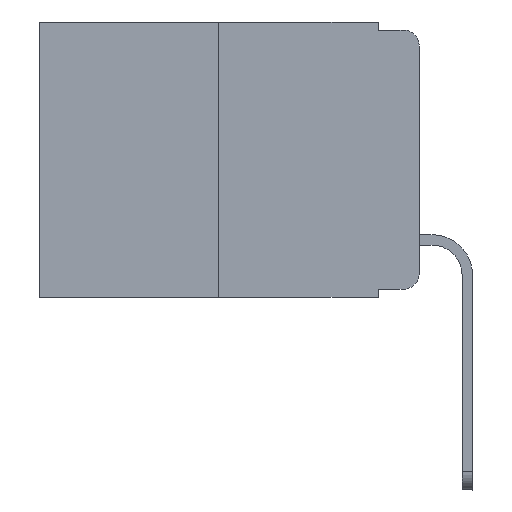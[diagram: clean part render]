
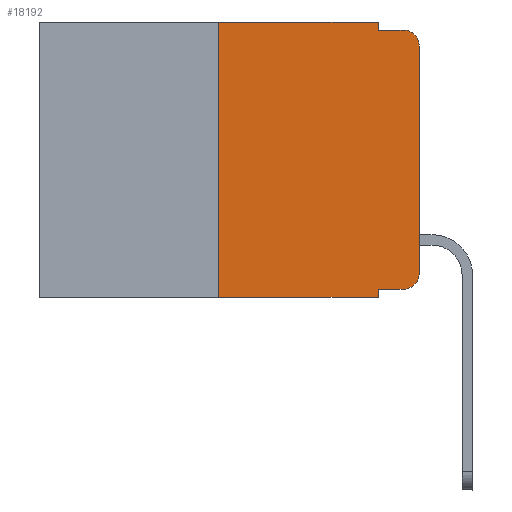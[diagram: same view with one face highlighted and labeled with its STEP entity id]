
A CAD part, left-side view. The second image highlights one B-rep face of the part: STEP entity #18192.
In plain terms, the highlighted planar face has unit normal (-1, 0, 0).
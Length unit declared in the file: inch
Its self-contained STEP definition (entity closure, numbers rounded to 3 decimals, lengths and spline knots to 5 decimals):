
#50 = ORIENTED_EDGE ( 'NONE', *, *, #8898, .F. ) ;
#95 = CARTESIAN_POINT ( 'NONE',  ( 0., 0.473, 0. ) ) ;
#233 = CARTESIAN_POINT ( 'NONE',  ( 0., 0.051, 0. ) ) ;
#463 = ORIENTED_EDGE ( 'NONE', *, *, #5389, .F. ) ;
#675 = ORIENTED_EDGE ( 'NONE', *, *, #1581, .T. ) ;
#876 = EDGE_CURVE ( 'NONE', #15493, #17174, #11914, .T. ) ;
#1025 = CARTESIAN_POINT ( 'NONE',  ( 0., 0.473, -0.343 ) ) ;
#1058 = EDGE_CURVE ( 'NONE', #11851, #17174, #5843, .T. ) ;
#1124 = ORIENTED_EDGE ( 'NONE', *, *, #15442, .F. ) ;
#1167 = DIRECTION ( 'NONE',  ( 0., 0., -1. ) ) ;
#1537 = LINE ( 'NONE', #95, #8032 ) ;
#1581 = EDGE_CURVE ( 'NONE', #4658, #11851, #10361, .T. ) ;
#1603 = DIRECTION ( 'NONE',  ( 0., -1., 0. ) ) ;
#1783 = EDGE_CURVE ( 'NONE', #18148, #4658, #7457, .T. ) ;
#1835 = DIRECTION ( 'NONE',  ( 0., 0., 1. ) ) ;
#1850 = LINE ( 'NONE', #7413, #16776 ) ;
#2966 = DIRECTION ( 'NONE',  ( 0., 0., -1. ) ) ;
#3089 = CARTESIAN_POINT ( 'NONE',  ( 0., 0., 0. ) ) ;
#3404 = CARTESIAN_POINT ( 'NONE',  ( 0., 0.051, -0.343 ) ) ;
#3584 = CARTESIAN_POINT ( 'NONE',  ( 0., 0.02, -0.03 ) ) ;
#3688 = DIRECTION ( 'NONE',  ( -1., 0., 0. ) ) ;
#3850 = ORIENTED_EDGE ( 'NONE', *, *, #876, .F. ) ;
#4001 = EDGE_CURVE ( 'NONE', #15682, #5826, #12594, .T. ) ;
#4401 = CARTESIAN_POINT ( 'NONE',  ( 0., 0.051, 0. ) ) ;
#4635 = AXIS2_PLACEMENT_3D ( 'NONE', #3584, #3688, #10580 ) ;
#4658 = VERTEX_POINT ( 'NONE', #16838 ) ;
#4681 = CARTESIAN_POINT ( 'NONE',  ( 0., 0.25, -0.343 ) ) ;
#4690 = AXIS2_PLACEMENT_3D ( 'NONE', #8340, #17420, #17240 ) ;
#4838 = CARTESIAN_POINT ( 'NONE',  ( 0., 0.25, 0. ) ) ;
#5173 = ORIENTED_EDGE ( 'NONE', *, *, #4001, .T. ) ;
#5241 = DIRECTION ( 'NONE',  ( 1., 0., 0. ) ) ;
#5389 = EDGE_CURVE ( 'NONE', #15682, #6582, #6472, .T. ) ;
#5418 = PLANE ( 'NONE',  #13416 ) ;
#5640 = CARTESIAN_POINT ( 'NONE',  ( 0., 0.051, -0.01 ) ) ;
#5826 = VERTEX_POINT ( 'NONE', #3404 ) ;
#5843 = CIRCLE ( 'NONE', #4635, 0.02 ) ;
#6472 = LINE ( 'NONE', #4838, #14893 ) ;
#6582 = VERTEX_POINT ( 'NONE', #14206 ) ;
#7400 = ORIENTED_EDGE ( 'NONE', *, *, #1058, .T. ) ;
#7413 = CARTESIAN_POINT ( 'NONE',  ( 0., 0.051, -0.333 ) ) ;
#7457 = CIRCLE ( 'NONE', #4690, 0.02 ) ;
#8032 = VECTOR ( 'NONE', #17147, 39.37008 ) ;
#8091 = VERTEX_POINT ( 'NONE', #233 ) ;
#8289 = ORIENTED_EDGE ( 'NONE', *, *, #1783, .T. ) ;
#8307 = VECTOR ( 'NONE', #1167, 39.37008 ) ;
#8340 = CARTESIAN_POINT ( 'NONE',  ( 0., 0.02, -0.313 ) ) ;
#8385 = DIRECTION ( 'NONE',  ( 0., -1., 0. ) ) ;
#8679 = CARTESIAN_POINT ( 'NONE',  ( 0., 0.051, -0.01 ) ) ;
#8717 = LINE ( 'NONE', #4401, #16402 ) ;
#8898 = EDGE_CURVE ( 'NONE', #15991, #5826, #18856, .T. ) ;
#9747 = CARTESIAN_POINT ( 'NONE',  ( 0., 0.473, 0. ) ) ;
#10361 = LINE ( 'NONE', #3089, #14350 ) ;
#10512 = CARTESIAN_POINT ( 'NONE',  ( 0., 0.051, -0.333 ) ) ;
#10551 = ORIENTED_EDGE ( 'NONE', *, *, #14223, .F. ) ;
#10580 = DIRECTION ( 'NONE',  ( 0., 0., -1. ) ) ;
#10690 = DIRECTION ( 'NONE',  ( 0., 0., 1. ) ) ;
#10989 = EDGE_LOOP ( 'NONE', ( #675, #7400, #3850, #1124, #10551, #463, #5173, #50, #18119, #8289 ) ) ;
#11088 = DIRECTION ( 'NONE',  ( 0., 0., -1. ) ) ;
#11380 = FACE_OUTER_BOUND ( 'NONE', #10989, .T. ) ;
#11766 = CARTESIAN_POINT ( 'NONE',  ( 0., 0.051, 0. ) ) ;
#11851 = VERTEX_POINT ( 'NONE', #13776 ) ;
#11914 = LINE ( 'NONE', #8679, #17743 ) ;
#11989 = DIRECTION ( 'NONE',  ( 0., -1., 0. ) ) ;
#12594 = LINE ( 'NONE', #1025, #15464 ) ;
#12695 = CARTESIAN_POINT ( 'NONE',  ( 0., 0.02, -0.333 ) ) ;
#13416 = AXIS2_PLACEMENT_3D ( 'NONE', #9747, #5241, #11088 ) ;
#13776 = CARTESIAN_POINT ( 'NONE',  ( 0., 0., -0.03 ) ) ;
#14206 = CARTESIAN_POINT ( 'NONE',  ( 0., 0.25, 0. ) ) ;
#14223 = EDGE_CURVE ( 'NONE', #6582, #8091, #1537, .T. ) ;
#14350 = VECTOR ( 'NONE', #1835, 39.37008 ) ;
#14893 = VECTOR ( 'NONE', #10690, 39.37008 ) ;
#15442 = EDGE_CURVE ( 'NONE', #8091, #15493, #8717, .T. ) ;
#15464 = VECTOR ( 'NONE', #8385, 39.37008 ) ;
#15493 = VERTEX_POINT ( 'NONE', #5640 ) ;
#15682 = VERTEX_POINT ( 'NONE', #4681 ) ;
#15991 = VERTEX_POINT ( 'NONE', #10512 ) ;
#16402 = VECTOR ( 'NONE', #2966, 39.37008 ) ;
#16776 = VECTOR ( 'NONE', #11989, 39.37008 ) ;
#16788 = EDGE_CURVE ( 'NONE', #15991, #18148, #1850, .T. ) ;
#16838 = CARTESIAN_POINT ( 'NONE',  ( 0., 0., -0.313 ) ) ;
#17147 = DIRECTION ( 'NONE',  ( 0., -1., 0. ) ) ;
#17174 = VERTEX_POINT ( 'NONE', #17684 ) ;
#17240 = DIRECTION ( 'NONE',  ( 0., 0., -1. ) ) ;
#17420 = DIRECTION ( 'NONE',  ( -1., 0., 0. ) ) ;
#17684 = CARTESIAN_POINT ( 'NONE',  ( 0., 0.02, -0.01 ) ) ;
#17743 = VECTOR ( 'NONE', #1603, 39.37008 ) ;
#18119 = ORIENTED_EDGE ( 'NONE', *, *, #16788, .T. ) ;
#18148 = VERTEX_POINT ( 'NONE', #12695 ) ;
#18192 = ADVANCED_FACE ( 'NONE', ( #11380 ), #5418, .F. ) ;
#18856 = LINE ( 'NONE', #11766, #8307 ) ;
